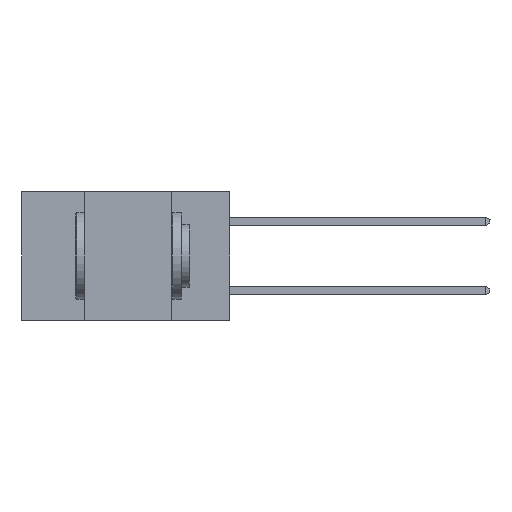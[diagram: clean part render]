
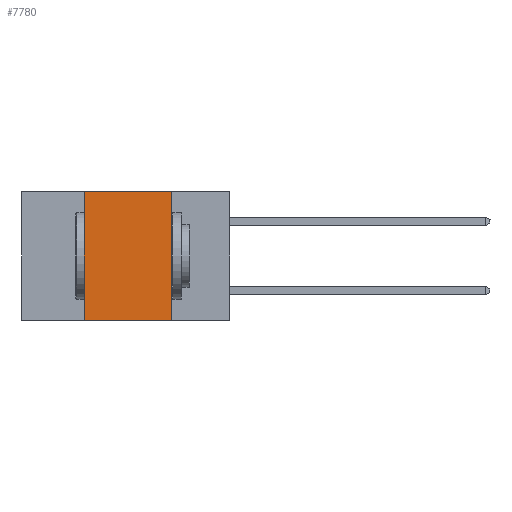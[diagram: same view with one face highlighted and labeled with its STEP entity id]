
A CAD part, left-side view. The second image highlights one B-rep face of the part: STEP entity #7780.
In plain terms, the highlighted planar face has unit normal (-1, 0, 0).
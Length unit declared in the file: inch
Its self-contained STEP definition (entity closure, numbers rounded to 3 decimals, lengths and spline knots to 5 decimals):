
#45 = VERTEX_POINT ( 'NONE', #21941 ) ;
#1170 = EDGE_CURVE ( 'NONE', #45, #24289, #15055, .T. ) ;
#1408 = ORIENTED_EDGE ( 'NONE', *, *, #26413, .T. ) ;
#2739 = CARTESIAN_POINT ( 'NONE',  ( 0., 0.42, 0. ) ) ;
#3025 = CARTESIAN_POINT ( 'NONE',  ( 0., 0.17, -0.37 ) ) ;
#5071 = DIRECTION ( 'NONE',  ( 0., 0., 1. ) ) ;
#5214 = LINE ( 'NONE', #5346, #12703 ) ;
#5346 = CARTESIAN_POINT ( 'NONE',  ( 0., 0.6, 0. ) ) ;
#5804 = DIRECTION ( 'NONE',  ( 0., -1., 0. ) ) ;
#5858 = VECTOR ( 'NONE', #12359, 39.37008 ) ;
#7550 = PLANE ( 'NONE',  #26117 ) ;
#7780 = ADVANCED_FACE ( 'NONE', ( #26505 ), #7550, .F. ) ;
#8621 = CARTESIAN_POINT ( 'NONE',  ( 0., 0.17, -0.37 ) ) ;
#9781 = DIRECTION ( 'NONE',  ( 0., -1., 0. ) ) ;
#9813 = EDGE_CURVE ( 'NONE', #23774, #10552, #16931, .T. ) ;
#10242 = LINE ( 'NONE', #24754, #17802 ) ;
#10270 = VECTOR ( 'NONE', #5071, 39.37008 ) ;
#10552 = VERTEX_POINT ( 'NONE', #3025 ) ;
#11568 = DIRECTION ( 'NONE',  ( 0., 0., -1. ) ) ;
#12359 = DIRECTION ( 'NONE',  ( 0., 0., -1. ) ) ;
#12703 = VECTOR ( 'NONE', #9781, 39.37008 ) ;
#13386 = CARTESIAN_POINT ( 'NONE',  ( 0., 0.42, -0.37 ) ) ;
#15055 = LINE ( 'NONE', #13386, #10270 ) ;
#16931 = LINE ( 'NONE', #8621, #5858 ) ;
#17802 = VECTOR ( 'NONE', #5804, 39.37008 ) ;
#19246 = EDGE_CURVE ( 'NONE', #24289, #23774, #5214, .T. ) ;
#21941 = CARTESIAN_POINT ( 'NONE',  ( 0., 0.42, -0.37 ) ) ;
#22146 = ORIENTED_EDGE ( 'NONE', *, *, #9813, .F. ) ;
#23375 = CARTESIAN_POINT ( 'NONE',  ( 0., 0.17, 0. ) ) ;
#23774 = VERTEX_POINT ( 'NONE', #23375 ) ;
#24102 = ORIENTED_EDGE ( 'NONE', *, *, #19246, .F. ) ;
#24164 = ORIENTED_EDGE ( 'NONE', *, *, #1170, .F. ) ;
#24289 = VERTEX_POINT ( 'NONE', #2739 ) ;
#24408 = CARTESIAN_POINT ( 'NONE',  ( 0., 0.6, 0. ) ) ;
#24754 = CARTESIAN_POINT ( 'NONE',  ( 0., 0.6, -0.37 ) ) ;
#26117 = AXIS2_PLACEMENT_3D ( 'NONE', #24408, #26648, #11568 ) ;
#26317 = EDGE_LOOP ( 'NONE', ( #22146, #24102, #24164, #1408 ) ) ;
#26413 = EDGE_CURVE ( 'NONE', #45, #10552, #10242, .T. ) ;
#26505 = FACE_OUTER_BOUND ( 'NONE', #26317, .T. ) ;
#26648 = DIRECTION ( 'NONE',  ( 1., 0., 0. ) ) ;
